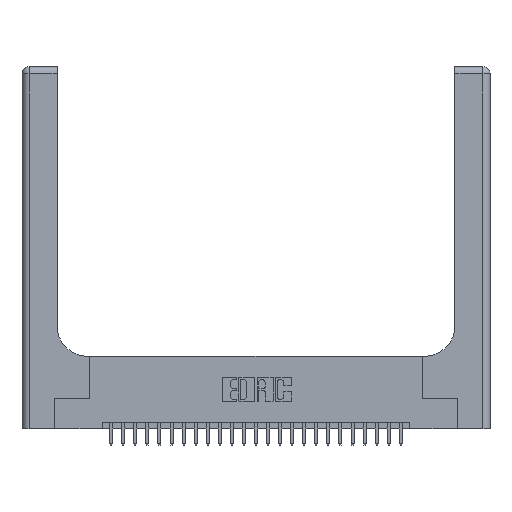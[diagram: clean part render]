
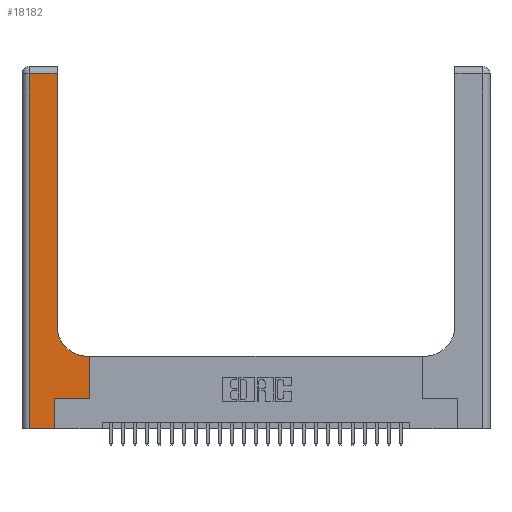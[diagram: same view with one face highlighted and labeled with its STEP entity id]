
A CAD part, top view. The second image highlights one B-rep face of the part: STEP entity #18182.
In plain terms, the highlighted planar face has unit normal (0, 0, 1).
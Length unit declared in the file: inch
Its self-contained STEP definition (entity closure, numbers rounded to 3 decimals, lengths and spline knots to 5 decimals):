
#1565 = VERTEX_POINT ( 'NONE', #16971 ) ;
#1769 = VERTEX_POINT ( 'NONE', #17942 ) ;
#1931 = CARTESIAN_POINT ( 'NONE',  ( 0.2915, 0.85, 0.37 ) ) ;
#1987 = CARTESIAN_POINT ( 'NONE',  ( 0., 2.94, 0.37 ) ) ;
#2012 = DIRECTION ( 'NONE',  ( 0., 0., -1. ) ) ;
#2475 = VECTOR ( 'NONE', #18630, 39.37008 ) ;
#4279 = DIRECTION ( 'NONE',  ( 0., 1., 0. ) ) ;
#5193 = ORIENTED_EDGE ( 'NONE', *, *, #26213, .T. ) ;
#5383 = DIRECTION ( 'NONE',  ( 1., 0., 0. ) ) ;
#5467 = EDGE_CURVE ( 'NONE', #1769, #14448, #10986, .T. ) ;
#5644 = VECTOR ( 'NONE', #13214, 39.37008 ) ;
#5731 = VECTOR ( 'NONE', #24985, 39.37008 ) ;
#5763 = CARTESIAN_POINT ( 'NONE',  ( 0.5585, 0.6, 0.37 ) ) ;
#5777 = ORIENTED_EDGE ( 'NONE', *, *, #16612, .T. ) ;
#5903 = EDGE_LOOP ( 'NONE', ( #27057, #12319, #26357, #21207, #8296, #5193, #5777, #11029, #9881 ) ) ;
#6174 = CARTESIAN_POINT ( 'NONE',  ( 0.269, 0.25, 0.37 ) ) ;
#6218 = CARTESIAN_POINT ( 'NONE',  ( 0.06, 3., 0.37 ) ) ;
#6513 = VERTEX_POINT ( 'NONE', #22943 ) ;
#7866 = CARTESIAN_POINT ( 'NONE',  ( 0.269, 0., 0.37 ) ) ;
#8296 = ORIENTED_EDGE ( 'NONE', *, *, #21665, .T. ) ;
#8903 = CARTESIAN_POINT ( 'NONE',  ( 0., 0., 0.37 ) ) ;
#9519 = CARTESIAN_POINT ( 'NONE',  ( 0.5415, 0.6, 0.37 ) ) ;
#9742 = LINE ( 'NONE', #16738, #16922 ) ;
#9787 = VECTOR ( 'NONE', #22401, 39.37008 ) ;
#9881 = ORIENTED_EDGE ( 'NONE', *, *, #12521, .T. ) ;
#9896 = CARTESIAN_POINT ( 'NONE',  ( 0.2915, 0.6, 0.37 ) ) ;
#9923 = AXIS2_PLACEMENT_3D ( 'NONE', #27015, #2012, #14498 ) ;
#10265 = DIRECTION ( 'NONE',  ( -1., 0., 0. ) ) ;
#10986 = LINE ( 'NONE', #6218, #5731 ) ;
#11029 = ORIENTED_EDGE ( 'NONE', *, *, #14550, .T. ) ;
#11589 = VECTOR ( 'NONE', #15679, 39.37008 ) ;
#11743 = LINE ( 'NONE', #26513, #9787 ) ;
#11824 = VERTEX_POINT ( 'NONE', #25929 ) ;
#11960 = CARTESIAN_POINT ( 'NONE',  ( 0.5415, 0.85, 0.37 ) ) ;
#12319 = ORIENTED_EDGE ( 'NONE', *, *, #13270, .T. ) ;
#12521 = EDGE_CURVE ( 'NONE', #19202, #18187, #14500, .T. ) ;
#12797 = LINE ( 'NONE', #1987, #19709 ) ;
#12845 = EDGE_CURVE ( 'NONE', #14448, #18705, #18410, .T. ) ;
#13214 = DIRECTION ( 'NONE',  ( 1., 0., 0. ) ) ;
#13270 = EDGE_CURVE ( 'NONE', #6513, #1769, #12797, .T. ) ;
#14103 = DIRECTION ( 'NONE',  ( 0., 0., -1. ) ) ;
#14448 = VERTEX_POINT ( 'NONE', #15766 ) ;
#14498 = DIRECTION ( 'NONE',  ( -1., 0., 0. ) ) ;
#14500 = CIRCLE ( 'NONE', #16344, 0.25 ) ;
#14550 = EDGE_CURVE ( 'NONE', #21883, #19202, #23221, .T. ) ;
#14590 = PLANE ( 'NONE',  #9923 ) ;
#14714 = VECTOR ( 'NONE', #26715, 39.37008 ) ;
#15035 = EDGE_CURVE ( 'NONE', #18187, #6513, #11743, .T. ) ;
#15679 = DIRECTION ( 'NONE',  ( 0., 1., 0. ) ) ;
#15766 = CARTESIAN_POINT ( 'NONE',  ( 0.06, 0., 0.37 ) ) ;
#16344 = AXIS2_PLACEMENT_3D ( 'NONE', #11960, #14103, #5383 ) ;
#16612 = EDGE_CURVE ( 'NONE', #1565, #21883, #9742, .T. ) ;
#16738 = CARTESIAN_POINT ( 'NONE',  ( 0.5585, 0.25, 0.37 ) ) ;
#16922 = VECTOR ( 'NONE', #4279, 39.37008 ) ;
#16971 = CARTESIAN_POINT ( 'NONE',  ( 0.5585, 0.25, 0.37 ) ) ;
#17942 = CARTESIAN_POINT ( 'NONE',  ( 0.06, 2.94, 0.37 ) ) ;
#18182 = ADVANCED_FACE ( 'NONE', ( #26990 ), #14590, .F. ) ;
#18187 = VERTEX_POINT ( 'NONE', #1931 ) ;
#18410 = LINE ( 'NONE', #8903, #5644 ) ;
#18630 = DIRECTION ( 'NONE',  ( 1., 0., 0. ) ) ;
#18705 = VERTEX_POINT ( 'NONE', #7866 ) ;
#19202 = VERTEX_POINT ( 'NONE', #9519 ) ;
#19688 = CARTESIAN_POINT ( 'NONE',  ( 0.269, 0., 0.37 ) ) ;
#19709 = VECTOR ( 'NONE', #10265, 39.37008 ) ;
#21207 = ORIENTED_EDGE ( 'NONE', *, *, #12845, .T. ) ;
#21665 = EDGE_CURVE ( 'NONE', #18705, #11824, #23067, .T. ) ;
#21883 = VERTEX_POINT ( 'NONE', #5763 ) ;
#22401 = DIRECTION ( 'NONE',  ( 0., 1., 0. ) ) ;
#22943 = CARTESIAN_POINT ( 'NONE',  ( 0.2915, 2.94, 0.37 ) ) ;
#23067 = LINE ( 'NONE', #19688, #11589 ) ;
#23221 = LINE ( 'NONE', #9896, #14714 ) ;
#24806 = LINE ( 'NONE', #6174, #2475 ) ;
#24985 = DIRECTION ( 'NONE',  ( 0., -1., 0. ) ) ;
#25929 = CARTESIAN_POINT ( 'NONE',  ( 0.269, 0.25, 0.37 ) ) ;
#26213 = EDGE_CURVE ( 'NONE', #11824, #1565, #24806, .T. ) ;
#26357 = ORIENTED_EDGE ( 'NONE', *, *, #5467, .T. ) ;
#26513 = CARTESIAN_POINT ( 'NONE',  ( 0.2915, 3., 0.37 ) ) ;
#26715 = DIRECTION ( 'NONE',  ( -1., 0., 0. ) ) ;
#26990 = FACE_OUTER_BOUND ( 'NONE', #5903, .T. ) ;
#27015 = CARTESIAN_POINT ( 'NONE',  ( 0., 3., 0.37 ) ) ;
#27057 = ORIENTED_EDGE ( 'NONE', *, *, #15035, .T. ) ;
